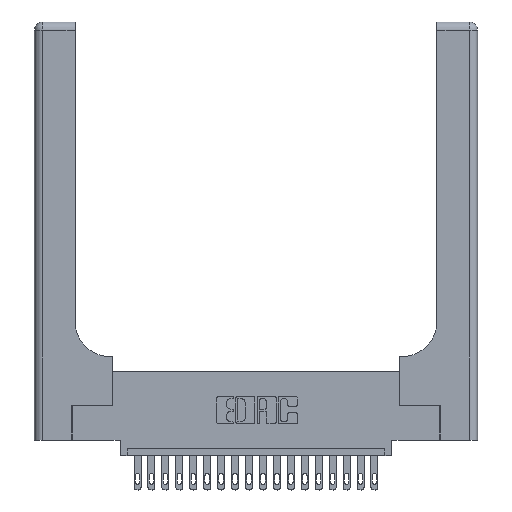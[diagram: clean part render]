
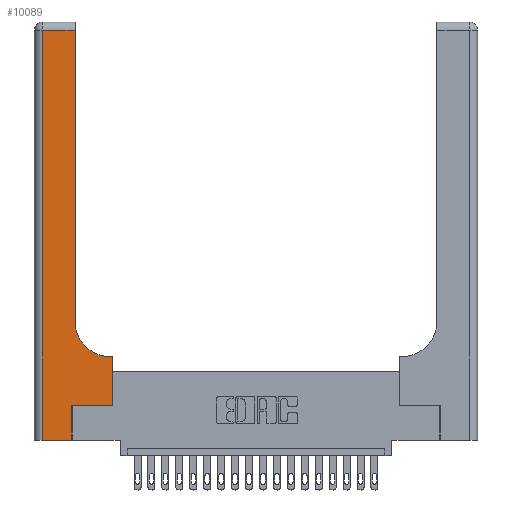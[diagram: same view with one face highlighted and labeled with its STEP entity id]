
A CAD part, top view. The second image highlights one B-rep face of the part: STEP entity #10089.
In plain terms, the highlighted planar face has unit normal (0, 0, 1).
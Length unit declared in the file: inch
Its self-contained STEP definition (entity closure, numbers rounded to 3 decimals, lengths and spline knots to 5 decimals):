
#1132 = LINE ( 'NONE', #7594, #17584 ) ;
#1337 = CARTESIAN_POINT ( 'NONE',  ( 0.2915, 2.94, 0.37 ) ) ;
#1530 = CARTESIAN_POINT ( 'NONE',  ( 0.2915, 0.85, 0.37 ) ) ;
#1845 = VERTEX_POINT ( 'NONE', #10777 ) ;
#2351 = LINE ( 'NONE', #16573, #19873 ) ;
#2439 = ORIENTED_EDGE ( 'NONE', *, *, #7597, .T. ) ;
#2462 = CARTESIAN_POINT ( 'NONE',  ( 0.06, 0., 0.37 ) ) ;
#3212 = EDGE_CURVE ( 'NONE', #4311, #17508, #6911, .T. ) ;
#3316 = EDGE_CURVE ( 'NONE', #4418, #4311, #10093, .T. ) ;
#3419 = DIRECTION ( 'NONE',  ( -1., 0., 0. ) ) ;
#3621 = CARTESIAN_POINT ( 'NONE',  ( 0.06, 3., 0.37 ) ) ;
#4311 = VERTEX_POINT ( 'NONE', #2462 ) ;
#4409 = LINE ( 'NONE', #6842, #19514 ) ;
#4418 = VERTEX_POINT ( 'NONE', #22002 ) ;
#4471 = DIRECTION ( 'NONE',  ( 0., 1., 0. ) ) ;
#4749 = DIRECTION ( 'NONE',  ( 0., 0., -1. ) ) ;
#4792 = DIRECTION ( 'NONE',  ( 0., 1., 0. ) ) ;
#5968 = CARTESIAN_POINT ( 'NONE',  ( 0.2915, 3., 0.37 ) ) ;
#6183 = ORIENTED_EDGE ( 'NONE', *, *, #18976, .T. ) ;
#6842 = CARTESIAN_POINT ( 'NONE',  ( 0., 2.94, 0.37 ) ) ;
#6911 = LINE ( 'NONE', #12553, #7464 ) ;
#7283 = EDGE_CURVE ( 'NONE', #21426, #15256, #11801, .T. ) ;
#7464 = VECTOR ( 'NONE', #14297, 39.37008 ) ;
#7501 = AXIS2_PLACEMENT_3D ( 'NONE', #8054, #4749, #13070 ) ;
#7572 = EDGE_LOOP ( 'NONE', ( #10301, #13241, #13260, #20702, #20633, #8679, #6183, #2439, #18709 ) ) ;
#7594 = CARTESIAN_POINT ( 'NONE',  ( 0.2915, 0.6, 0.37 ) ) ;
#7597 = EDGE_CURVE ( 'NONE', #21899, #21948, #1132, .T. ) ;
#8054 = CARTESIAN_POINT ( 'NONE',  ( 0.5415, 0.85, 0.37 ) ) ;
#8160 = CARTESIAN_POINT ( 'NONE',  ( 0.5585, 0.6, 0.37 ) ) ;
#8679 = ORIENTED_EDGE ( 'NONE', *, *, #13236, .T. ) ;
#9160 = VERTEX_POINT ( 'NONE', #10748 ) ;
#9645 = CARTESIAN_POINT ( 'NONE',  ( 0.269, 0., 0.37 ) ) ;
#9938 = CARTESIAN_POINT ( 'NONE',  ( 0.5415, 0.6, 0.37 ) ) ;
#9971 = LINE ( 'NONE', #18300, #20567 ) ;
#10089 = ADVANCED_FACE ( 'NONE', ( #18502 ), #20787, .F. ) ;
#10093 = LINE ( 'NONE', #3621, #18812 ) ;
#10301 = ORIENTED_EDGE ( 'NONE', *, *, #7283, .T. ) ;
#10418 = DIRECTION ( 'NONE',  ( 0., 0., -1. ) ) ;
#10748 = CARTESIAN_POINT ( 'NONE',  ( 0.5585, 0.25, 0.37 ) ) ;
#10777 = CARTESIAN_POINT ( 'NONE',  ( 0.269, 0.25, 0.37 ) ) ;
#10789 = AXIS2_PLACEMENT_3D ( 'NONE', #18904, #10418, #15713 ) ;
#10942 = VECTOR ( 'NONE', #15168, 39.37008 ) ;
#11436 = EDGE_CURVE ( 'NONE', #15256, #4418, #4409, .T. ) ;
#11801 = LINE ( 'NONE', #5968, #15739 ) ;
#11939 = DIRECTION ( 'NONE',  ( 0., -1., 0. ) ) ;
#12004 = CARTESIAN_POINT ( 'NONE',  ( 0.5585, 0.25, 0.37 ) ) ;
#12553 = CARTESIAN_POINT ( 'NONE',  ( 0., 0., 0.37 ) ) ;
#12763 = DIRECTION ( 'NONE',  ( -1., 0., 0. ) ) ;
#12997 = DIRECTION ( 'NONE',  ( 1., 0., 0. ) ) ;
#13070 = DIRECTION ( 'NONE',  ( 1., 0., 0. ) ) ;
#13236 = EDGE_CURVE ( 'NONE', #1845, #9160, #9971, .T. ) ;
#13241 = ORIENTED_EDGE ( 'NONE', *, *, #11436, .T. ) ;
#13260 = ORIENTED_EDGE ( 'NONE', *, *, #3316, .T. ) ;
#13979 = CIRCLE ( 'NONE', #7501, 0.25 ) ;
#14297 = DIRECTION ( 'NONE',  ( 1., 0., 0. ) ) ;
#15168 = DIRECTION ( 'NONE',  ( 0., 1., 0. ) ) ;
#15256 = VERTEX_POINT ( 'NONE', #1337 ) ;
#15713 = DIRECTION ( 'NONE',  ( -1., 0., 0. ) ) ;
#15739 = VECTOR ( 'NONE', #4471, 39.37008 ) ;
#15935 = LINE ( 'NONE', #12004, #10942 ) ;
#16491 = EDGE_CURVE ( 'NONE', #17508, #1845, #2351, .T. ) ;
#16573 = CARTESIAN_POINT ( 'NONE',  ( 0.269, 0., 0.37 ) ) ;
#17508 = VERTEX_POINT ( 'NONE', #9645 ) ;
#17584 = VECTOR ( 'NONE', #12763, 39.37008 ) ;
#18195 = EDGE_CURVE ( 'NONE', #21948, #21426, #13979, .T. ) ;
#18300 = CARTESIAN_POINT ( 'NONE',  ( 0.269, 0.25, 0.37 ) ) ;
#18502 = FACE_OUTER_BOUND ( 'NONE', #7572, .T. ) ;
#18709 = ORIENTED_EDGE ( 'NONE', *, *, #18195, .T. ) ;
#18812 = VECTOR ( 'NONE', #11939, 39.37008 ) ;
#18904 = CARTESIAN_POINT ( 'NONE',  ( 0., 3., 0.37 ) ) ;
#18976 = EDGE_CURVE ( 'NONE', #9160, #21899, #15935, .T. ) ;
#19514 = VECTOR ( 'NONE', #3419, 39.37008 ) ;
#19873 = VECTOR ( 'NONE', #4792, 39.37008 ) ;
#20567 = VECTOR ( 'NONE', #12997, 39.37008 ) ;
#20633 = ORIENTED_EDGE ( 'NONE', *, *, #16491, .T. ) ;
#20702 = ORIENTED_EDGE ( 'NONE', *, *, #3212, .T. ) ;
#20787 = PLANE ( 'NONE',  #10789 ) ;
#21426 = VERTEX_POINT ( 'NONE', #1530 ) ;
#21899 = VERTEX_POINT ( 'NONE', #8160 ) ;
#21948 = VERTEX_POINT ( 'NONE', #9938 ) ;
#22002 = CARTESIAN_POINT ( 'NONE',  ( 0.06, 2.94, 0.37 ) ) ;
